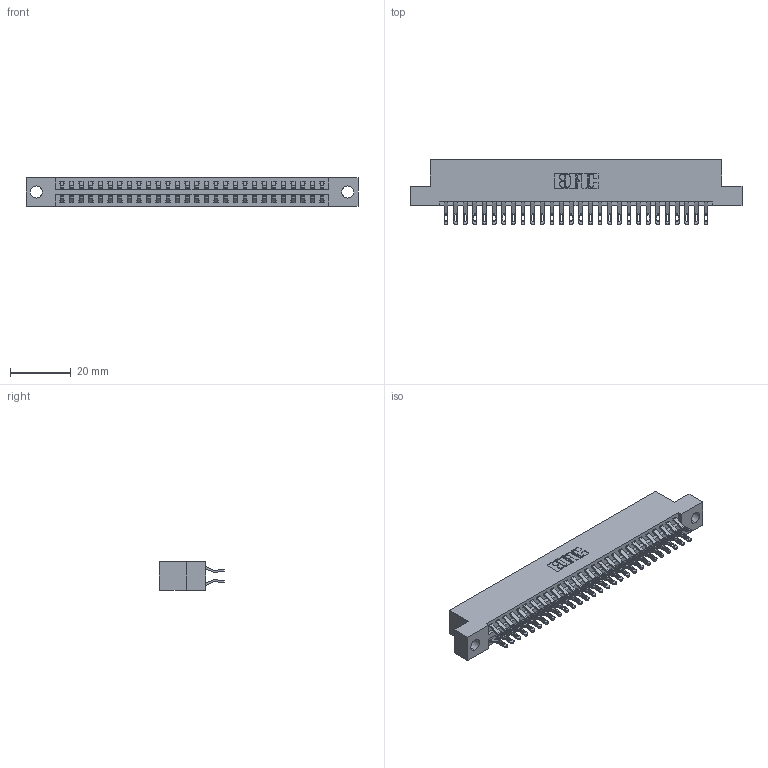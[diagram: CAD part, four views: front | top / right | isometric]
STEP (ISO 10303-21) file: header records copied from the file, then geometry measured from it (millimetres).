
FILE_DESCRIPTION (( 'STEP AP203' ), '1' );
FILE_NAME ('346-056-555-204.STEP', '2022-05-21T06:14:43', ( '' ), ( '' ), 'SwSTEP 2.0', 'SolidWorks 2020', '' );
FILE_SCHEMA (( 'CONFIG_CONTROL_DESIGN' ));
Length unit declared in the file: inch
Products named in the file (3): 345-292-001_555 Tail; 346-056-555-204; 346 Part_Flush Mounting Lugs - 0.156 Dia-TH
Assembly tree (57 placements, depth 2):
  346-056-555-204
    346 Part_Flush Mounting Lugs - 0.156 Dia-TH
    345-292-001_555 Tail  x56
Bounding box: 109.47 x 21.46 x 9.4 mm (x, y, z)
Volume: 10622.8 mm3; surface area: 14808.6 mm2
Topology: 57 solids, 57 shells, 3384 faces, 10613 edges, 7074 vertices
Faces by surface type: plane 1938, cylinder 1446
Entity records: 20903 total; most frequent: CARTESIAN_POINT 3504, ORIENTED_EDGE 3406, DIRECTION 3107, EDGE_CURVE 1703, LINE 1439, VECTOR 1439, VERTEX_POINT 1134, AXIS2_PLACEMENT_3D 834
